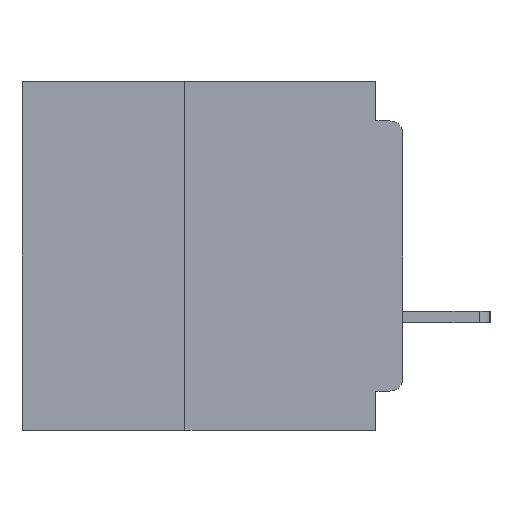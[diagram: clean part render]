
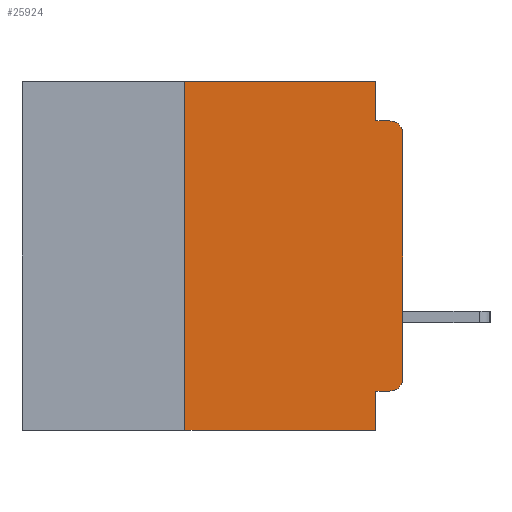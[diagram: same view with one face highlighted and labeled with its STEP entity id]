
A CAD part, left-side view. The second image highlights one B-rep face of the part: STEP entity #25924.
In plain terms, the highlighted planar face has unit normal (-1, 0, 0).
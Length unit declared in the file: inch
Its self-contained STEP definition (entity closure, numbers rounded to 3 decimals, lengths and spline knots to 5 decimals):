
#774 = LINE ( 'NONE', #3424, #43288 ) ;
#1882 = DIRECTION ( 'NONE',  ( 0., -1., 0. ) ) ;
#2332 = DIRECTION ( 'NONE',  ( 0., -1., 0. ) ) ;
#2739 = CARTESIAN_POINT ( 'NONE',  ( 0., 0.031, 0. ) ) ;
#2962 = ORIENTED_EDGE ( 'NONE', *, *, #20500, .F. ) ;
#3424 = CARTESIAN_POINT ( 'NONE',  ( 0., 0.031, 0. ) ) ;
#4959 = ORIENTED_EDGE ( 'NONE', *, *, #37432, .F. ) ;
#5816 = CARTESIAN_POINT ( 'NONE',  ( 0., 0.031, -0.4 ) ) ;
#6077 = CARTESIAN_POINT ( 'NONE',  ( 0., 0., -0.045 ) ) ;
#7234 = CARTESIAN_POINT ( 'NONE',  ( 0., 0., -0.355 ) ) ;
#9060 = ORIENTED_EDGE ( 'NONE', *, *, #27005, .F. ) ;
#9355 = CARTESIAN_POINT ( 'NONE',  ( 0., 0., -0.06 ) ) ;
#10626 = CARTESIAN_POINT ( 'NONE',  ( 0., 0.015, -0.06 ) ) ;
#10962 = LINE ( 'NONE', #7234, #54358 ) ;
#11067 = CARTESIAN_POINT ( 'NONE',  ( 0., 0.015, -0.045 ) ) ;
#11296 = LINE ( 'NONE', #19492, #54671 ) ;
#12129 = DIRECTION ( 'NONE',  ( 0., 0., -1. ) ) ;
#13024 = VERTEX_POINT ( 'NONE', #9355 ) ;
#13362 = VERTEX_POINT ( 'NONE', #53656 ) ;
#13640 = LINE ( 'NONE', #19612, #34891 ) ;
#14689 = LINE ( 'NONE', #25381, #37192 ) ;
#14975 = DIRECTION ( 'NONE',  ( 0., 0., -1. ) ) ;
#15711 = DIRECTION ( 'NONE',  ( -1., 0., 0. ) ) ;
#16519 = ORIENTED_EDGE ( 'NONE', *, *, #27316, .T. ) ;
#17148 = EDGE_LOOP ( 'NONE', ( #45941, #34339, #49236, #4959, #9060, #2962, #16519, #21880, #46712, #25943 ) ) ;
#17332 = CARTESIAN_POINT ( 'NONE',  ( 0., 0.25, -0.4 ) ) ;
#17363 = EDGE_CURVE ( 'NONE', #13024, #51658, #20936, .T. ) ;
#19492 = CARTESIAN_POINT ( 'NONE',  ( 0., 0.437, -0.4 ) ) ;
#19612 = CARTESIAN_POINT ( 'NONE',  ( 0., 0.031, -0.4 ) ) ;
#20500 = EDGE_CURVE ( 'NONE', #46676, #13362, #50122, .T. ) ;
#20734 = VERTEX_POINT ( 'NONE', #5816 ) ;
#20936 = CIRCLE ( 'NONE', #22278, 0.015 ) ;
#21379 = PLANE ( 'NONE',  #53688 ) ;
#21700 = CARTESIAN_POINT ( 'NONE',  ( 0., 0.031, -0.045 ) ) ;
#21732 = DIRECTION ( 'NONE',  ( 0., 0., -1. ) ) ;
#21815 = VERTEX_POINT ( 'NONE', #21700 ) ;
#21880 = ORIENTED_EDGE ( 'NONE', *, *, #24470, .F. ) ;
#22278 = AXIS2_PLACEMENT_3D ( 'NONE', #10626, #40188, #14975 ) ;
#23507 = CARTESIAN_POINT ( 'NONE',  ( 0., 0., 0. ) ) ;
#24470 = EDGE_CURVE ( 'NONE', #43181, #20734, #13640, .T. ) ;
#25381 = CARTESIAN_POINT ( 'NONE',  ( 0., 0.437, 0. ) ) ;
#25924 = ADVANCED_FACE ( 'NONE', ( #28235 ), #21379, .F. ) ;
#25943 = ORIENTED_EDGE ( 'NONE', *, *, #43732, .T. ) ;
#26531 = VECTOR ( 'NONE', #1882, 39.37008 ) ;
#27005 = EDGE_CURVE ( 'NONE', #13362, #35991, #14689, .T. ) ;
#27316 = EDGE_CURVE ( 'NONE', #46676, #20734, #11296, .T. ) ;
#28235 = FACE_OUTER_BOUND ( 'NONE', #17148, .T. ) ;
#28528 = EDGE_CURVE ( 'NONE', #40745, #13024, #29236, .T. ) ;
#28793 = DIRECTION ( 'NONE',  ( 0., 1., 0. ) ) ;
#29236 = LINE ( 'NONE', #23507, #37650 ) ;
#29576 = EDGE_CURVE ( 'NONE', #21815, #51658, #48610, .T. ) ;
#32191 = DIRECTION ( 'NONE',  ( 0., 0., 1. ) ) ;
#32814 = CARTESIAN_POINT ( 'NONE',  ( 0., 0., -0.34 ) ) ;
#33054 = CARTESIAN_POINT ( 'NONE',  ( 0., 0.015, -0.355 ) ) ;
#34339 = ORIENTED_EDGE ( 'NONE', *, *, #17363, .T. ) ;
#34891 = VECTOR ( 'NONE', #44688, 39.37008 ) ;
#35884 = CARTESIAN_POINT ( 'NONE',  ( 0., 0.25, -0.4 ) ) ;
#35991 = VERTEX_POINT ( 'NONE', #2739 ) ;
#36040 = VERTEX_POINT ( 'NONE', #33054 ) ;
#37192 = VECTOR ( 'NONE', #54441, 39.37008 ) ;
#37432 = EDGE_CURVE ( 'NONE', #35991, #21815, #774, .T. ) ;
#37650 = VECTOR ( 'NONE', #32191, 39.37008 ) ;
#37920 = AXIS2_PLACEMENT_3D ( 'NONE', #40895, #15711, #45045 ) ;
#38355 = DIRECTION ( 'NONE',  ( 0., 0., 1. ) ) ;
#39048 = VECTOR ( 'NONE', #38355, 39.37008 ) ;
#40188 = DIRECTION ( 'NONE',  ( -1., 0., 0. ) ) ;
#40259 = CIRCLE ( 'NONE', #37920, 0.015 ) ;
#40745 = VERTEX_POINT ( 'NONE', #32814 ) ;
#40895 = CARTESIAN_POINT ( 'NONE',  ( 0., 0.015, -0.34 ) ) ;
#41315 = CARTESIAN_POINT ( 'NONE',  ( 0., 0.031, -0.355 ) ) ;
#42558 = CARTESIAN_POINT ( 'NONE',  ( 0., 0.437, 0. ) ) ;
#43181 = VERTEX_POINT ( 'NONE', #41315 ) ;
#43288 = VECTOR ( 'NONE', #12129, 39.37008 ) ;
#43732 = EDGE_CURVE ( 'NONE', #36040, #40745, #40259, .T. ) ;
#44688 = DIRECTION ( 'NONE',  ( 0., 0., -1. ) ) ;
#45045 = DIRECTION ( 'NONE',  ( 0., 0., -1. ) ) ;
#45475 = EDGE_CURVE ( 'NONE', #36040, #43181, #10962, .T. ) ;
#45941 = ORIENTED_EDGE ( 'NONE', *, *, #28528, .T. ) ;
#46676 = VERTEX_POINT ( 'NONE', #35884 ) ;
#46712 = ORIENTED_EDGE ( 'NONE', *, *, #45475, .F. ) ;
#46744 = DIRECTION ( 'NONE',  ( 1., 0., 0. ) ) ;
#48610 = LINE ( 'NONE', #6077, #26531 ) ;
#49236 = ORIENTED_EDGE ( 'NONE', *, *, #29576, .F. ) ;
#50122 = LINE ( 'NONE', #17332, #39048 ) ;
#51658 = VERTEX_POINT ( 'NONE', #11067 ) ;
#53656 = CARTESIAN_POINT ( 'NONE',  ( 0., 0.25, 0. ) ) ;
#53688 = AXIS2_PLACEMENT_3D ( 'NONE', #42558, #46744, #21732 ) ;
#54358 = VECTOR ( 'NONE', #28793, 39.37008 ) ;
#54441 = DIRECTION ( 'NONE',  ( 0., -1., 0. ) ) ;
#54671 = VECTOR ( 'NONE', #2332, 39.37008 ) ;
